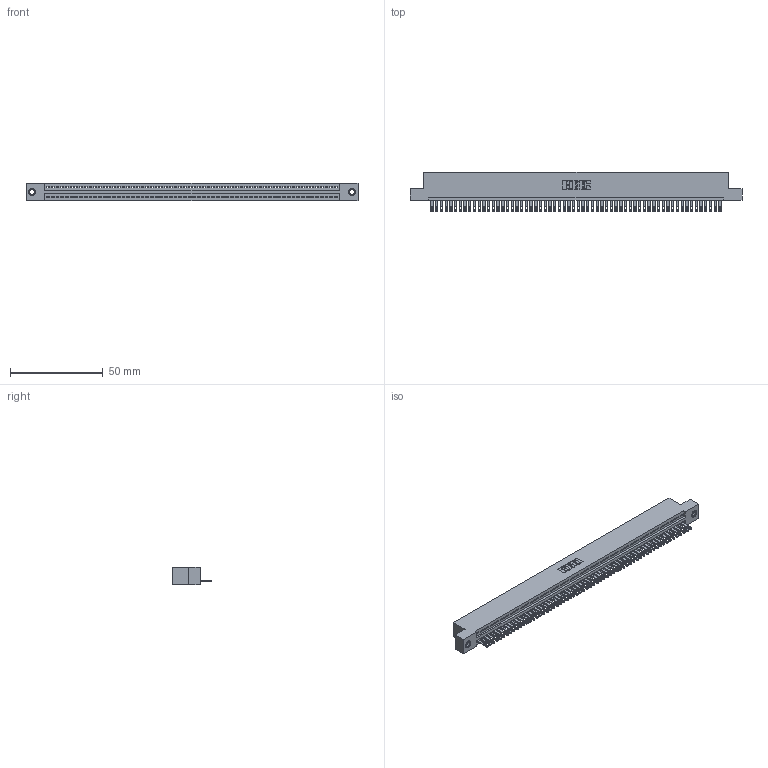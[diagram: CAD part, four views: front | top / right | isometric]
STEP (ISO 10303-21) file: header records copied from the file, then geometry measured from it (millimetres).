
FILE_DESCRIPTION (( 'STEP AP203' ), '1' );
FILE_NAME ('345-062-500-107.STEP', '2019-10-11T04:05:57', ( '' ), ( '' ), 'SwSTEP 2.0', 'SolidWorks 2016', '' );
FILE_SCHEMA (( 'CONFIG_CONTROL_DESIGN' ));
Length unit declared in the file: inch
Products named in the file (4): 345-250-001_345-250-005-103; 345-062-500-107; 345-292-001_345-293-100; 345 Part_Flush Mounting Lugs - 0.156 Dia-TI
Assembly tree (65 placements, depth 2):
  345-062-500-107
    345 Part_Flush Mounting Lugs - 0.156 Dia-TI
    345-292-001_345-293-100  x62
    345-250-001_345-250-005-103  x2
Bounding box: 178.69 x 21.51 x 9.4 mm (x, y, z)
Volume: 17160.8 mm3; surface area: 23248.7 mm2
Topology: 65 solids, 65 shells, 3534 faces, 10893 edges, 7254 vertices
Faces by surface type: plane 2220, cylinder 1298, cone 12, torus 4
Entity records: 45086 total; most frequent: CARTESIAN_POINT 7789, ORIENTED_EDGE 7778, DIRECTION 6803, EDGE_CURVE 3889, LINE 3485, VECTOR 3485, VERTEX_POINT 2588, AXIS2_PLACEMENT_3D 1659
